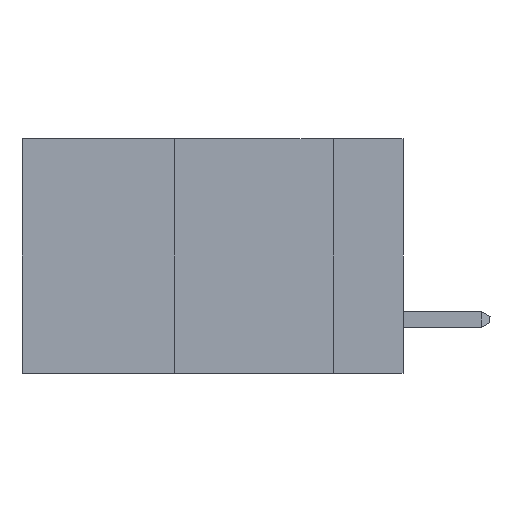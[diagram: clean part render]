
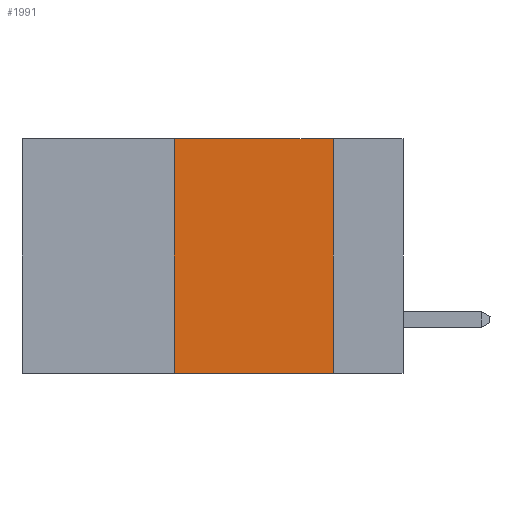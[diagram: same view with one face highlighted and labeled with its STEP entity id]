
A CAD part, left-side view. The second image highlights one B-rep face of the part: STEP entity #1991.
In plain terms, the highlighted planar face has unit normal (-1, 0, 0).
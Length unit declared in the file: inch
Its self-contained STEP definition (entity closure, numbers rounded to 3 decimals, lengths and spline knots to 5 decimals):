
#1991 = ADVANCED_FACE ( 'NONE', ( #7020 ), #3421, .F. ) ;
#2031 = CARTESIAN_POINT ( 'NONE',  ( 0., 0.11, 0. ) ) ;
#2106 = VERTEX_POINT ( 'NONE', #12029 ) ;
#2568 = CARTESIAN_POINT ( 'NONE',  ( 0., 0.36, -0.37 ) ) ;
#3421 = PLANE ( 'NONE',  #4685 ) ;
#3631 = EDGE_CURVE ( 'NONE', #19246, #11013, #12776, .T. ) ;
#3950 = DIRECTION ( 'NONE',  ( 0., 0., -1. ) ) ;
#4685 = AXIS2_PLACEMENT_3D ( 'NONE', #8950, #15366, #9078 ) ;
#4828 = DIRECTION ( 'NONE',  ( 0., -1., 0. ) ) ;
#5630 = ORIENTED_EDGE ( 'NONE', *, *, #3631, .F. ) ;
#6260 = LINE ( 'NONE', #2031, #16249 ) ;
#6752 = ORIENTED_EDGE ( 'NONE', *, *, #11220, .F. ) ;
#7020 = FACE_OUTER_BOUND ( 'NONE', #25217, .T. ) ;
#7355 = LINE ( 'NONE', #9046, #14357 ) ;
#8494 = CARTESIAN_POINT ( 'NONE',  ( 0., 0.6, -0.37 ) ) ;
#8950 = CARTESIAN_POINT ( 'NONE',  ( 0., 0.6, 0. ) ) ;
#9046 = CARTESIAN_POINT ( 'NONE',  ( 0., 0.36, 0. ) ) ;
#9078 = DIRECTION ( 'NONE',  ( 0., 0., -1. ) ) ;
#10390 = CARTESIAN_POINT ( 'NONE',  ( 0., 0.36, 0. ) ) ;
#10681 = DIRECTION ( 'NONE',  ( 0., -1., 0. ) ) ;
#10696 = CARTESIAN_POINT ( 'NONE',  ( 0., 0.11, 0. ) ) ;
#11013 = VERTEX_POINT ( 'NONE', #10696 ) ;
#11220 = EDGE_CURVE ( 'NONE', #11013, #2106, #6260, .T. ) ;
#12029 = CARTESIAN_POINT ( 'NONE',  ( 0., 0.11, -0.37 ) ) ;
#12551 = VERTEX_POINT ( 'NONE', #2568 ) ;
#12776 = LINE ( 'NONE', #22037, #16784 ) ;
#13895 = LINE ( 'NONE', #8494, #15165 ) ;
#14266 = ORIENTED_EDGE ( 'NONE', *, *, #23716, .F. ) ;
#14357 = VECTOR ( 'NONE', #14950, 39.37008 ) ;
#14950 = DIRECTION ( 'NONE',  ( 0., 0., 1. ) ) ;
#15165 = VECTOR ( 'NONE', #10681, 39.37008 ) ;
#15366 = DIRECTION ( 'NONE',  ( 1., 0., 0. ) ) ;
#16249 = VECTOR ( 'NONE', #3950, 39.37008 ) ;
#16784 = VECTOR ( 'NONE', #4828, 39.37008 ) ;
#17306 = EDGE_CURVE ( 'NONE', #12551, #2106, #13895, .T. ) ;
#19246 = VERTEX_POINT ( 'NONE', #10390 ) ;
#19278 = ORIENTED_EDGE ( 'NONE', *, *, #17306, .T. ) ;
#22037 = CARTESIAN_POINT ( 'NONE',  ( 0., 0.6, 0. ) ) ;
#23716 = EDGE_CURVE ( 'NONE', #12551, #19246, #7355, .T. ) ;
#25217 = EDGE_LOOP ( 'NONE', ( #6752, #5630, #14266, #19278 ) ) ;
